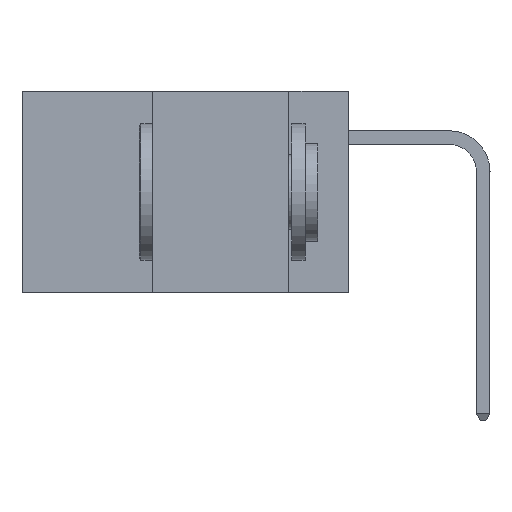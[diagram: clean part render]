
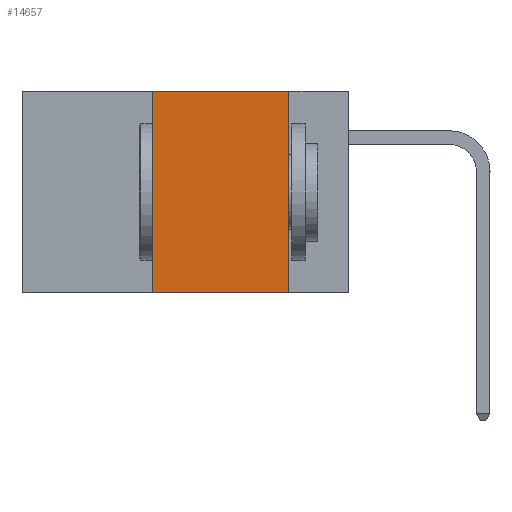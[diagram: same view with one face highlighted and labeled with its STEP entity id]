
A CAD part, left-side view. The second image highlights one B-rep face of the part: STEP entity #14657.
In plain terms, the highlighted planar face has unit normal (-1, 0, 0).
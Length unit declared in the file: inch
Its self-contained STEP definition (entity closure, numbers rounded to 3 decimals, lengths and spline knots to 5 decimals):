
#164 = DIRECTION ( 'NONE',  ( 0., -1., 0. ) ) ;
#1363 = EDGE_CURVE ( 'NONE', #5526, #11680, #37471, .T. ) ;
#2559 = ORIENTED_EDGE ( 'NONE', *, *, #18128, .T. ) ;
#5201 = CARTESIAN_POINT ( 'NONE',  ( 0., 0.11, -0.37 ) ) ;
#5526 = VERTEX_POINT ( 'NONE', #28928 ) ;
#6054 = DIRECTION ( 'NONE',  ( 0., -1., 0. ) ) ;
#8236 = CARTESIAN_POINT ( 'NONE',  ( 0., 0.6, 0. ) ) ;
#9174 = CARTESIAN_POINT ( 'NONE',  ( 0., 0.6, 0. ) ) ;
#9202 = VECTOR ( 'NONE', #164, 39.37008 ) ;
#10154 = LINE ( 'NONE', #12363, #34141 ) ;
#11057 = EDGE_CURVE ( 'NONE', #11680, #27010, #10154, .T. ) ;
#11530 = DIRECTION ( 'NONE',  ( 0., 0., -1. ) ) ;
#11680 = VERTEX_POINT ( 'NONE', #21934 ) ;
#12363 = CARTESIAN_POINT ( 'NONE',  ( 0., 0.11, 0. ) ) ;
#12480 = EDGE_CURVE ( 'NONE', #31361, #5526, #39193, .T. ) ;
#13283 = CARTESIAN_POINT ( 'NONE',  ( 0., 0.6, -0.37 ) ) ;
#14279 = CARTESIAN_POINT ( 'NONE',  ( 0., 0.36, -0.37 ) ) ;
#14657 = ADVANCED_FACE ( 'NONE', ( #35916 ), #34225, .F. ) ;
#16983 = ORIENTED_EDGE ( 'NONE', *, *, #1363, .F. ) ;
#18128 = EDGE_CURVE ( 'NONE', #31361, #27010, #26623, .T. ) ;
#19851 = VECTOR ( 'NONE', #26554, 39.37008 ) ;
#19919 = EDGE_LOOP ( 'NONE', ( #36595, #16983, #26548, #2559 ) ) ;
#21934 = CARTESIAN_POINT ( 'NONE',  ( 0., 0.11, 0. ) ) ;
#23289 = CARTESIAN_POINT ( 'NONE',  ( 0., 0.36, 0. ) ) ;
#24869 = AXIS2_PLACEMENT_3D ( 'NONE', #8236, #31060, #11530 ) ;
#26548 = ORIENTED_EDGE ( 'NONE', *, *, #12480, .F. ) ;
#26554 = DIRECTION ( 'NONE',  ( 0., 0., 1. ) ) ;
#26623 = LINE ( 'NONE', #13283, #9202 ) ;
#27010 = VERTEX_POINT ( 'NONE', #5201 ) ;
#28815 = VECTOR ( 'NONE', #6054, 39.37008 ) ;
#28928 = CARTESIAN_POINT ( 'NONE',  ( 0., 0.36, 0. ) ) ;
#31060 = DIRECTION ( 'NONE',  ( 1., 0., 0. ) ) ;
#31361 = VERTEX_POINT ( 'NONE', #14279 ) ;
#34141 = VECTOR ( 'NONE', #38446, 39.37008 ) ;
#34225 = PLANE ( 'NONE',  #24869 ) ;
#35916 = FACE_OUTER_BOUND ( 'NONE', #19919, .T. ) ;
#36595 = ORIENTED_EDGE ( 'NONE', *, *, #11057, .F. ) ;
#37471 = LINE ( 'NONE', #9174, #28815 ) ;
#38446 = DIRECTION ( 'NONE',  ( 0., 0., -1. ) ) ;
#39193 = LINE ( 'NONE', #23289, #19851 ) ;
